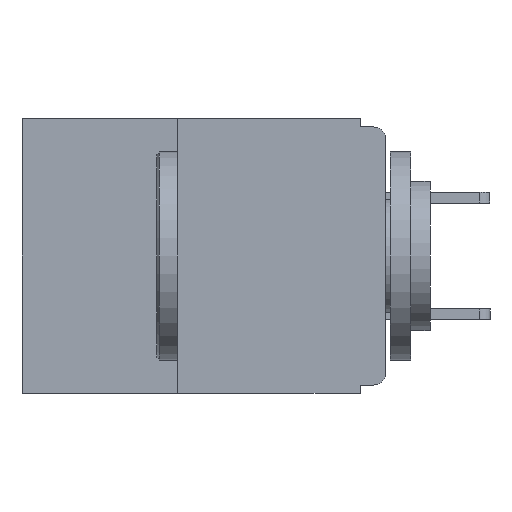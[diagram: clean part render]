
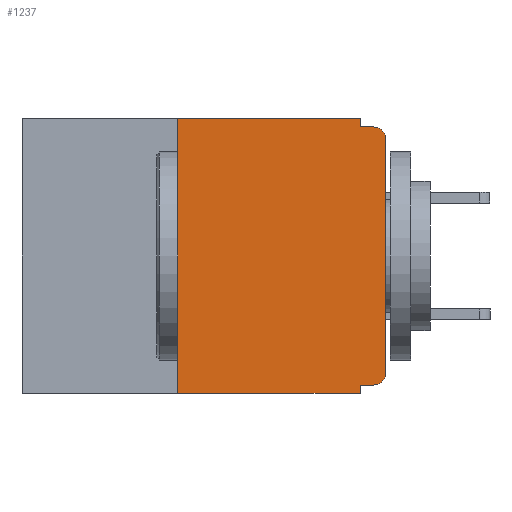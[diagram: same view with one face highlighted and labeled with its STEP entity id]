
A CAD part, left-side view. The second image highlights one B-rep face of the part: STEP entity #1237.
In plain terms, the highlighted planar face has unit normal (-1, 0, 0).
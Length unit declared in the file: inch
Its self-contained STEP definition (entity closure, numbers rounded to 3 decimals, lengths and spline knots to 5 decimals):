
#996 = DIRECTION ( 'NONE',  ( 0., 1., 0. ) ) ;
#1237 = ADVANCED_FACE ( 'NONE', ( #4659 ), #16166, .F. ) ;
#2058 = CARTESIAN_POINT ( 'NONE',  ( 0., 0.031, -0.33 ) ) ;
#2136 = LINE ( 'NONE', #4519, #20910 ) ;
#2159 = ORIENTED_EDGE ( 'NONE', *, *, #4031, .F. ) ;
#2175 = ORIENTED_EDGE ( 'NONE', *, *, #13566, .T. ) ;
#2516 = CIRCLE ( 'NONE', #10785, 0.015 ) ;
#2802 = CARTESIAN_POINT ( 'NONE',  ( 0., 0., 0. ) ) ;
#3584 = VERTEX_POINT ( 'NONE', #29486 ) ;
#4031 = EDGE_CURVE ( 'NONE', #8518, #28742, #21701, .T. ) ;
#4094 = VERTEX_POINT ( 'NONE', #21551 ) ;
#4519 = CARTESIAN_POINT ( 'NONE',  ( 0., 0.437, 0. ) ) ;
#4659 = FACE_OUTER_BOUND ( 'NONE', #28530, .T. ) ;
#4800 = CARTESIAN_POINT ( 'NONE',  ( 0., 0.437, -0.33 ) ) ;
#5018 = DIRECTION ( 'NONE',  ( 0., 0., -1. ) ) ;
#5080 = DIRECTION ( 'NONE',  ( 1., 0., 0. ) ) ;
#5271 = VERTEX_POINT ( 'NONE', #2058 ) ;
#5311 = DIRECTION ( 'NONE',  ( 0., 0., 1. ) ) ;
#6071 = CARTESIAN_POINT ( 'NONE',  ( 0., 0.25, -0.33 ) ) ;
#6480 = EDGE_CURVE ( 'NONE', #29849, #5271, #17907, .T. ) ;
#7255 = DIRECTION ( 'NONE',  ( 0., -1., 0. ) ) ;
#7362 = CARTESIAN_POINT ( 'NONE',  ( 0., 0.015, -0.305 ) ) ;
#7573 = LINE ( 'NONE', #4800, #24599 ) ;
#7989 = LINE ( 'NONE', #15233, #14205 ) ;
#8040 = EDGE_CURVE ( 'NONE', #17189, #5271, #7573, .T. ) ;
#8426 = CARTESIAN_POINT ( 'NONE',  ( 0., 0.015, -0.025 ) ) ;
#8518 = VERTEX_POINT ( 'NONE', #29679 ) ;
#8655 = VECTOR ( 'NONE', #22710, 39.37008 ) ;
#8816 = CARTESIAN_POINT ( 'NONE',  ( 0., 0.031, -0.32 ) ) ;
#9458 = VECTOR ( 'NONE', #16480, 39.37008 ) ;
#9713 = DIRECTION ( 'NONE',  ( 0., 0., -1. ) ) ;
#9798 = AXIS2_PLACEMENT_3D ( 'NONE', #22622, #5080, #5018 ) ;
#10472 = VERTEX_POINT ( 'NONE', #14065 ) ;
#10785 = AXIS2_PLACEMENT_3D ( 'NONE', #8426, #24611, #10787 ) ;
#10787 = DIRECTION ( 'NONE',  ( 0., 0., -1. ) ) ;
#10835 = CARTESIAN_POINT ( 'NONE',  ( 0., 0.25, -0.33 ) ) ;
#11213 = EDGE_CURVE ( 'NONE', #17189, #4094, #28353, .T. ) ;
#11617 = DIRECTION ( 'NONE',  ( 0., 0., -1. ) ) ;
#11797 = VECTOR ( 'NONE', #11617, 39.37008 ) ;
#11868 = CARTESIAN_POINT ( 'NONE',  ( 0., 0.031, 0. ) ) ;
#12277 = CARTESIAN_POINT ( 'NONE',  ( 0., 0.031, -0.33 ) ) ;
#12752 = EDGE_CURVE ( 'NONE', #10472, #8518, #27916, .T. ) ;
#13566 = EDGE_CURVE ( 'NONE', #21942, #22281, #23890, .T. ) ;
#14065 = CARTESIAN_POINT ( 'NONE',  ( 0., 0.031, 0. ) ) ;
#14146 = EDGE_CURVE ( 'NONE', #3584, #21942, #29037, .T. ) ;
#14205 = VECTOR ( 'NONE', #996, 39.37008 ) ;
#14481 = CARTESIAN_POINT ( 'NONE',  ( 0., 0., -0.025 ) ) ;
#15233 = CARTESIAN_POINT ( 'NONE',  ( 0., 0., -0.32 ) ) ;
#16166 = PLANE ( 'NONE',  #9798 ) ;
#16480 = DIRECTION ( 'NONE',  ( 0., 0., -1. ) ) ;
#17188 = EDGE_CURVE ( 'NONE', #22281, #28742, #2516, .T. ) ;
#17189 = VERTEX_POINT ( 'NONE', #6071 ) ;
#17404 = EDGE_CURVE ( 'NONE', #4094, #10472, #2136, .T. ) ;
#17778 = DIRECTION ( 'NONE',  ( 0., 0., 1. ) ) ;
#17907 = LINE ( 'NONE', #12277, #11797 ) ;
#18994 = ORIENTED_EDGE ( 'NONE', *, *, #8040, .T. ) ;
#19072 = ORIENTED_EDGE ( 'NONE', *, *, #6480, .F. ) ;
#19492 = ORIENTED_EDGE ( 'NONE', *, *, #14146, .T. ) ;
#20200 = AXIS2_PLACEMENT_3D ( 'NONE', #7362, #23570, #9713 ) ;
#20880 = DIRECTION ( 'NONE',  ( 0., -1., 0. ) ) ;
#20910 = VECTOR ( 'NONE', #20880, 39.37008 ) ;
#21501 = VECTOR ( 'NONE', #17778, 39.37008 ) ;
#21551 = CARTESIAN_POINT ( 'NONE',  ( 0., 0.25, 0. ) ) ;
#21701 = LINE ( 'NONE', #22277, #8655 ) ;
#21942 = VERTEX_POINT ( 'NONE', #23446 ) ;
#22248 = ORIENTED_EDGE ( 'NONE', *, *, #24953, .F. ) ;
#22277 = CARTESIAN_POINT ( 'NONE',  ( 0., 0., -0.01 ) ) ;
#22281 = VERTEX_POINT ( 'NONE', #14481 ) ;
#22622 = CARTESIAN_POINT ( 'NONE',  ( 0., 0.437, 0. ) ) ;
#22710 = DIRECTION ( 'NONE',  ( 0., -1., 0. ) ) ;
#23446 = CARTESIAN_POINT ( 'NONE',  ( 0., 0., -0.305 ) ) ;
#23547 = CARTESIAN_POINT ( 'NONE',  ( 0., 0.015, -0.01 ) ) ;
#23570 = DIRECTION ( 'NONE',  ( -1., 0., 0. ) ) ;
#23890 = LINE ( 'NONE', #2802, #28686 ) ;
#24137 = ORIENTED_EDGE ( 'NONE', *, *, #17404, .F. ) ;
#24599 = VECTOR ( 'NONE', #7255, 39.37008 ) ;
#24611 = DIRECTION ( 'NONE',  ( -1., 0., 0. ) ) ;
#24953 = EDGE_CURVE ( 'NONE', #3584, #29849, #7989, .T. ) ;
#25858 = ORIENTED_EDGE ( 'NONE', *, *, #11213, .F. ) ;
#27916 = LINE ( 'NONE', #11868, #9458 ) ;
#28353 = LINE ( 'NONE', #10835, #21501 ) ;
#28530 = EDGE_LOOP ( 'NONE', ( #2175, #29602, #2159, #29414, #24137, #25858, #18994, #19072, #22248, #19492 ) ) ;
#28686 = VECTOR ( 'NONE', #5311, 39.37008 ) ;
#28742 = VERTEX_POINT ( 'NONE', #23547 ) ;
#29037 = CIRCLE ( 'NONE', #20200, 0.015 ) ;
#29414 = ORIENTED_EDGE ( 'NONE', *, *, #12752, .F. ) ;
#29486 = CARTESIAN_POINT ( 'NONE',  ( 0., 0.015, -0.32 ) ) ;
#29602 = ORIENTED_EDGE ( 'NONE', *, *, #17188, .T. ) ;
#29679 = CARTESIAN_POINT ( 'NONE',  ( 0., 0.031, -0.01 ) ) ;
#29849 = VERTEX_POINT ( 'NONE', #8816 ) ;
